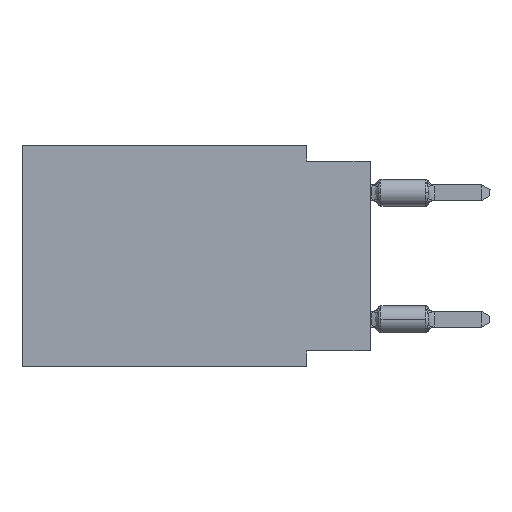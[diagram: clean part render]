
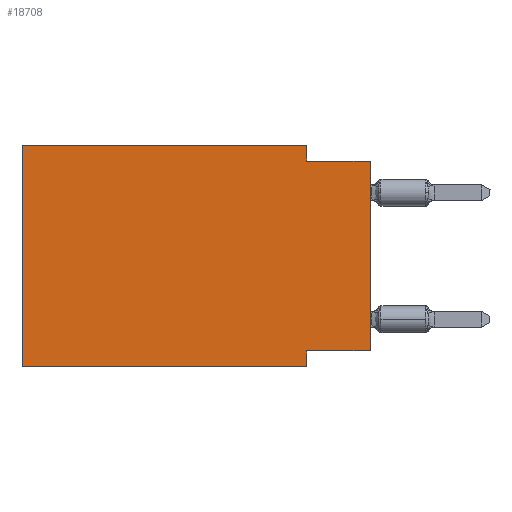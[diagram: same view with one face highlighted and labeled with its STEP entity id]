
A CAD part, left-side view. The second image highlights one B-rep face of the part: STEP entity #18708.
In plain terms, the highlighted planar face has unit normal (-1, 0, 0).
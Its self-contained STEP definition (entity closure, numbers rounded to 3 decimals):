
#2484 = VERTEX_POINT ( 'NONE', #15381 ) ;
#3427 = DIRECTION ( 'NONE',  ( 0., 0., 1. ) ) ;
#4686 = CARTESIAN_POINT ( 'NONE',  ( 0., 2.54, 0. ) ) ;
#5546 = EDGE_CURVE ( 'NONE', #24890, #31706, #29039, .T. ) ;
#5819 = ORIENTED_EDGE ( 'NONE', *, *, #38941, .F. ) ;
#5945 = DIRECTION ( 'NONE',  ( 0., 1., 0. ) ) ;
#6153 = LINE ( 'NONE', #33376, #23590 ) ;
#6647 = CARTESIAN_POINT ( 'NONE',  ( 0., 13.97, 0. ) ) ;
#7462 = CARTESIAN_POINT ( 'NONE',  ( 0., 2.54, -8.89 ) ) ;
#9152 = ORIENTED_EDGE ( 'NONE', *, *, #23080, .F. ) ;
#9283 = CARTESIAN_POINT ( 'NONE',  ( 0., 13.97, -8.89 ) ) ;
#9915 = CARTESIAN_POINT ( 'NONE',  ( 0., 2.54, -0.635 ) ) ;
#10048 = LINE ( 'NONE', #32151, #15819 ) ;
#10197 = EDGE_CURVE ( 'NONE', #29579, #26731, #34542, .T. ) ;
#11401 = VECTOR ( 'NONE', #22904, 1000. ) ;
#12236 = CARTESIAN_POINT ( 'NONE',  ( 0., 0., 0. ) ) ;
#12614 = EDGE_CURVE ( 'NONE', #2484, #26731, #14894, .T. ) ;
#13297 = CARTESIAN_POINT ( 'NONE',  ( 0., 13.97, 0. ) ) ;
#13620 = PLANE ( 'NONE',  #25074 ) ;
#13831 = DIRECTION ( 'NONE',  ( 1., 0., 0. ) ) ;
#14213 = LINE ( 'NONE', #39369, #14552 ) ;
#14552 = VECTOR ( 'NONE', #30371, 1000. ) ;
#14766 = DIRECTION ( 'NONE',  ( 0., 0., -1. ) ) ;
#14894 = LINE ( 'NONE', #12236, #29186 ) ;
#15217 = VECTOR ( 'NONE', #14766, 1000. ) ;
#15371 = EDGE_LOOP ( 'NONE', ( #40029, #17724, #5819, #20085, #30886, #24724, #28386, #9152 ) ) ;
#15381 = CARTESIAN_POINT ( 'NONE',  ( 0., 0., -8.255 ) ) ;
#15819 = VECTOR ( 'NONE', #19869, 1000. ) ;
#16115 = VERTEX_POINT ( 'NONE', #7462 ) ;
#16440 = VERTEX_POINT ( 'NONE', #9283 ) ;
#17479 = EDGE_CURVE ( 'NONE', #16440, #16115, #14213, .T. ) ;
#17724 = ORIENTED_EDGE ( 'NONE', *, *, #10197, .F. ) ;
#18017 = EDGE_CURVE ( 'NONE', #19723, #16115, #18240, .T. ) ;
#18240 = LINE ( 'NONE', #33779, #15217 ) ;
#18708 = ADVANCED_FACE ( 'NONE', ( #38772 ), #13620, .F. ) ;
#19723 = VERTEX_POINT ( 'NONE', #32947 ) ;
#19869 = DIRECTION ( 'NONE',  ( 0., 0., -1. ) ) ;
#20085 = ORIENTED_EDGE ( 'NONE', *, *, #5546, .F. ) ;
#20198 = DIRECTION ( 'NONE',  ( 0., -1., 0. ) ) ;
#20564 = CARTESIAN_POINT ( 'NONE',  ( 0., 13.97, 0. ) ) ;
#21871 = EDGE_CURVE ( 'NONE', #16440, #24890, #34521, .T. ) ;
#22279 = CARTESIAN_POINT ( 'NONE',  ( 0., 0., -0.635 ) ) ;
#22904 = DIRECTION ( 'NONE',  ( 0., -1., 0. ) ) ;
#22970 = CARTESIAN_POINT ( 'NONE',  ( 0., 0., -0.635 ) ) ;
#23080 = EDGE_CURVE ( 'NONE', #2484, #19723, #6153, .T. ) ;
#23590 = VECTOR ( 'NONE', #5945, 1000. ) ;
#24714 = CARTESIAN_POINT ( 'NONE',  ( 0., 13.97, 0. ) ) ;
#24724 = ORIENTED_EDGE ( 'NONE', *, *, #17479, .T. ) ;
#24890 = VERTEX_POINT ( 'NONE', #6647 ) ;
#25074 = AXIS2_PLACEMENT_3D ( 'NONE', #20564, #13831, #38959 ) ;
#26731 = VERTEX_POINT ( 'NONE', #22970 ) ;
#28386 = ORIENTED_EDGE ( 'NONE', *, *, #18017, .F. ) ;
#29039 = LINE ( 'NONE', #13297, #11401 ) ;
#29186 = VECTOR ( 'NONE', #37395, 1000. ) ;
#29579 = VERTEX_POINT ( 'NONE', #9915 ) ;
#30371 = DIRECTION ( 'NONE',  ( 0., -1., 0. ) ) ;
#30886 = ORIENTED_EDGE ( 'NONE', *, *, #21871, .F. ) ;
#31003 = VECTOR ( 'NONE', #3427, 1000. ) ;
#31706 = VERTEX_POINT ( 'NONE', #4686 ) ;
#32151 = CARTESIAN_POINT ( 'NONE',  ( 0., 2.54, 0. ) ) ;
#32947 = CARTESIAN_POINT ( 'NONE',  ( 0., 2.54, -8.255 ) ) ;
#33376 = CARTESIAN_POINT ( 'NONE',  ( 0., 0., -8.255 ) ) ;
#33779 = CARTESIAN_POINT ( 'NONE',  ( 0., 2.54, -8.89 ) ) ;
#34521 = LINE ( 'NONE', #24714, #31003 ) ;
#34542 = LINE ( 'NONE', #22279, #35276 ) ;
#35276 = VECTOR ( 'NONE', #20198, 1000. ) ;
#37395 = DIRECTION ( 'NONE',  ( 0., 0., 1. ) ) ;
#38772 = FACE_OUTER_BOUND ( 'NONE', #15371, .T. ) ;
#38941 = EDGE_CURVE ( 'NONE', #31706, #29579, #10048, .T. ) ;
#38959 = DIRECTION ( 'NONE',  ( 0., 0., -1. ) ) ;
#39369 = CARTESIAN_POINT ( 'NONE',  ( 0., 13.97, -8.89 ) ) ;
#40029 = ORIENTED_EDGE ( 'NONE', *, *, #12614, .T. ) ;
